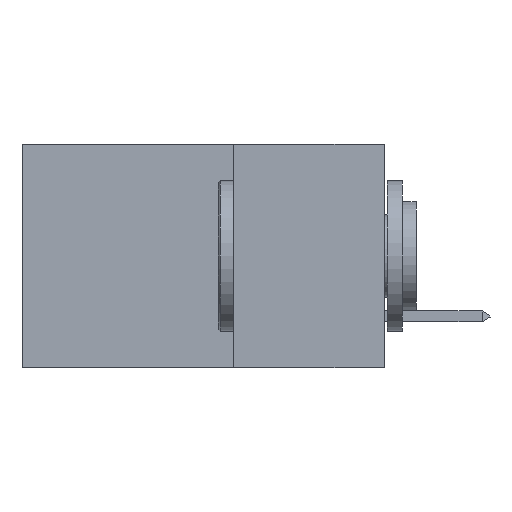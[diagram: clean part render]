
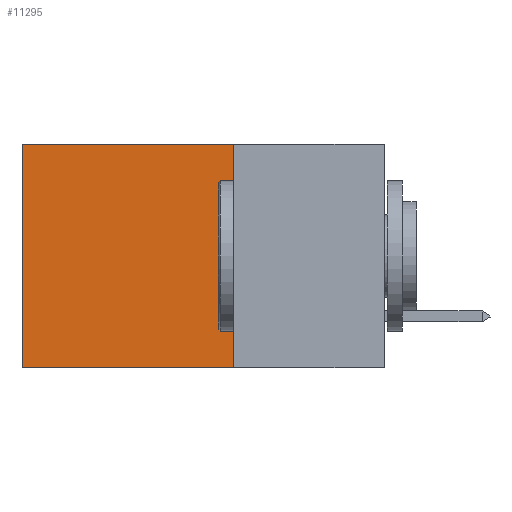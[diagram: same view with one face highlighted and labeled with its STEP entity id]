
A CAD part, left-side view. The second image highlights one B-rep face of the part: STEP entity #11295.
In plain terms, the highlighted planar face has unit normal (-1, 0, 0).
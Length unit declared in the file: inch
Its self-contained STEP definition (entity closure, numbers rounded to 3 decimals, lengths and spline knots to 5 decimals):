
#750 = CARTESIAN_POINT ( 'NONE',  ( 0.2875, 0.25, 0. ) ) ;
#793 = ORIENTED_EDGE ( 'NONE', *, *, #17230, .F. ) ;
#899 = CARTESIAN_POINT ( 'NONE',  ( 0.2875, 0.25, -0.37 ) ) ;
#1927 = DIRECTION ( 'NONE',  ( 0., 1., 0. ) ) ;
#2077 = CARTESIAN_POINT ( 'NONE',  ( 0.2875, 0.25, 0. ) ) ;
#2222 = DIRECTION ( 'NONE',  ( 0., 0., -1. ) ) ;
#2692 = CARTESIAN_POINT ( 'NONE',  ( 0.2875, 0.6, 0. ) ) ;
#3922 = LINE ( 'NONE', #2692, #13585 ) ;
#4351 = LINE ( 'NONE', #750, #7402 ) ;
#4357 = DIRECTION ( 'NONE',  ( 0., 1., 0. ) ) ;
#5925 = EDGE_LOOP ( 'NONE', ( #16504, #793, #31989, #17736 ) ) ;
#7402 = VECTOR ( 'NONE', #4357, 39.37008 ) ;
#7447 = DIRECTION ( 'NONE',  ( 1., 0., 0. ) ) ;
#8901 = VERTEX_POINT ( 'NONE', #10773 ) ;
#10717 = EDGE_CURVE ( 'NONE', #29095, #12417, #38612, .T. ) ;
#10773 = CARTESIAN_POINT ( 'NONE',  ( 0.2875, 0.6, -0.37 ) ) ;
#11295 = ADVANCED_FACE ( 'NONE', ( #32443 ), #21188, .F. ) ;
#12417 = VERTEX_POINT ( 'NONE', #27939 ) ;
#13585 = VECTOR ( 'NONE', #32346, 39.37008 ) ;
#16189 = EDGE_CURVE ( 'NONE', #26420, #8901, #3922, .T. ) ;
#16504 = ORIENTED_EDGE ( 'NONE', *, *, #16189, .T. ) ;
#17230 = EDGE_CURVE ( 'NONE', #12417, #8901, #31961, .T. ) ;
#17728 = CARTESIAN_POINT ( 'NONE',  ( 0.2875, 0.25, 0. ) ) ;
#17736 = ORIENTED_EDGE ( 'NONE', *, *, #24298, .T. ) ;
#21188 = PLANE ( 'NONE',  #38787 ) ;
#24298 = EDGE_CURVE ( 'NONE', #29095, #26420, #4351, .T. ) ;
#24468 = CARTESIAN_POINT ( 'NONE',  ( 0.2875, 0.25, 0. ) ) ;
#24852 = VECTOR ( 'NONE', #1927, 39.37008 ) ;
#26420 = VERTEX_POINT ( 'NONE', #40867 ) ;
#27939 = CARTESIAN_POINT ( 'NONE',  ( 0.2875, 0.25, -0.37 ) ) ;
#29095 = VERTEX_POINT ( 'NONE', #17728 ) ;
#31961 = LINE ( 'NONE', #899, #24852 ) ;
#31989 = ORIENTED_EDGE ( 'NONE', *, *, #10717, .F. ) ;
#32346 = DIRECTION ( 'NONE',  ( 0., 0., -1. ) ) ;
#32443 = FACE_OUTER_BOUND ( 'NONE', #5925, .T. ) ;
#38612 = LINE ( 'NONE', #2077, #40623 ) ;
#38787 = AXIS2_PLACEMENT_3D ( 'NONE', #24468, #7447, #2222 ) ;
#40623 = VECTOR ( 'NONE', #42176, 39.37008 ) ;
#40867 = CARTESIAN_POINT ( 'NONE',  ( 0.2875, 0.6, 0. ) ) ;
#42176 = DIRECTION ( 'NONE',  ( 0., 0., -1. ) ) ;
